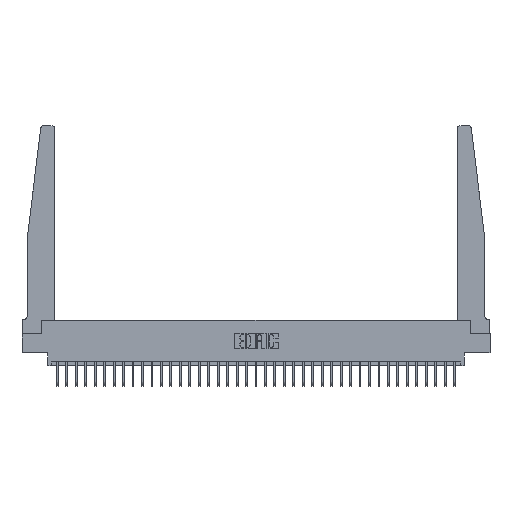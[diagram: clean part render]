
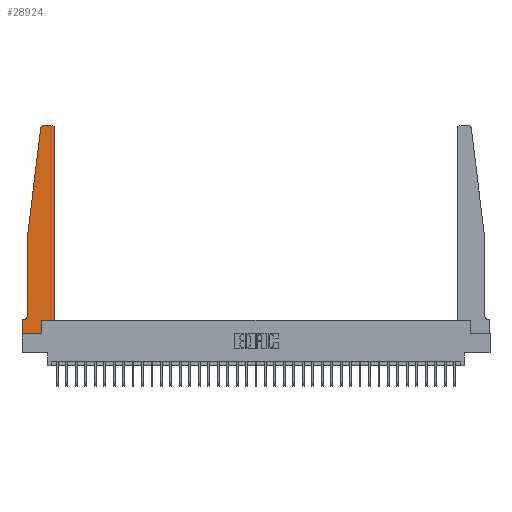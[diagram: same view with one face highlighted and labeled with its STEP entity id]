
A CAD part, top view. The second image highlights one B-rep face of the part: STEP entity #28924.
In plain terms, the highlighted planar face has unit normal (0, 0, 1).
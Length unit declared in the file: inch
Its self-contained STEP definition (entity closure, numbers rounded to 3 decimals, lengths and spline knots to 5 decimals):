
#155 = LINE ( 'NONE', #34775, #7327 ) ;
#225 = CARTESIAN_POINT ( 'NONE',  ( 0.27653, 2.72, 0.37 ) ) ;
#571 = CARTESIAN_POINT ( 'NONE',  ( 0.425, 0.18, 0.37 ) ) ;
#936 = VERTEX_POINT ( 'NONE', #23370 ) ;
#950 = CARTESIAN_POINT ( 'NONE',  ( 0.065, 1.25, 0.37 ) ) ;
#1851 = EDGE_CURVE ( 'NONE', #7147, #11979, #5981, .T. ) ;
#1907 = DIRECTION ( 'NONE',  ( 1., 0., 0. ) ) ;
#2014 = LINE ( 'NONE', #4502, #15001 ) ;
#2184 = VECTOR ( 'NONE', #29237, 39.37008 ) ;
#2485 = EDGE_CURVE ( 'NONE', #4802, #4737, #7721, .T. ) ;
#2605 = LINE ( 'NONE', #24413, #2184 ) ;
#3345 = CARTESIAN_POINT ( 'NONE',  ( 0.24675, 2.72367, 0.37 ) ) ;
#3614 = ORIENTED_EDGE ( 'NONE', *, *, #10190, .T. ) ;
#3928 = EDGE_CURVE ( 'NONE', #13896, #4141, #4807, .T. ) ;
#3960 = CARTESIAN_POINT ( 'NONE',  ( 0., 0.1875, 0.37 ) ) ;
#3990 = DIRECTION ( 'NONE',  ( 1., 0., 0. ) ) ;
#4141 = VERTEX_POINT ( 'NONE', #5384 ) ;
#4457 = EDGE_CURVE ( 'NONE', #21417, #7147, #25244, .T. ) ;
#4487 = CARTESIAN_POINT ( 'NONE',  ( 0.25, 2.75, 0.37 ) ) ;
#4502 = CARTESIAN_POINT ( 'NONE',  ( 0., 0., 0.37 ) ) ;
#4632 = EDGE_CURVE ( 'NONE', #936, #11196, #155, .T. ) ;
#4737 = VERTEX_POINT ( 'NONE', #3345 ) ;
#4747 = LINE ( 'NONE', #20705, #18385 ) ;
#4802 = VERTEX_POINT ( 'NONE', #26220 ) ;
#4807 = CIRCLE ( 'NONE', #7709, 0.03 ) ;
#5384 = CARTESIAN_POINT ( 'NONE',  ( 0.395, 2.75, 0.37 ) ) ;
#5981 = CIRCLE ( 'NONE', #29217, 0.05 ) ;
#6317 = CARTESIAN_POINT ( 'NONE',  ( 0.065, 0.1875, 0.37 ) ) ;
#7110 = FACE_OUTER_BOUND ( 'NONE', #29035, .T. ) ;
#7147 = VERTEX_POINT ( 'NONE', #27066 ) ;
#7327 = VECTOR ( 'NONE', #10977, 39.37008 ) ;
#7356 = CARTESIAN_POINT ( 'NONE',  ( 0.425, 0.18, 0.37 ) ) ;
#7709 = AXIS2_PLACEMENT_3D ( 'NONE', #28301, #19953, #3990 ) ;
#7721 = CIRCLE ( 'NONE', #27564, 0.03 ) ;
#7745 = DIRECTION ( 'NONE',  ( -0.122, -0.992, 0. ) ) ;
#8095 = CARTESIAN_POINT ( 'NONE',  ( 0.2605, 0.18, 0.37 ) ) ;
#8152 = ORIENTED_EDGE ( 'NONE', *, *, #18287, .T. ) ;
#8573 = DIRECTION ( 'NONE',  ( 0., 0., 1. ) ) ;
#8608 = DIRECTION ( 'NONE',  ( 0., -1., 0. ) ) ;
#9162 = DIRECTION ( 'NONE',  ( -1., 0., 0. ) ) ;
#10190 = EDGE_CURVE ( 'NONE', #4141, #4802, #28793, .T. ) ;
#10977 = DIRECTION ( 'NONE',  ( 0., 1., 0. ) ) ;
#11060 = EDGE_CURVE ( 'NONE', #4737, #21417, #4747, .T. ) ;
#11196 = VERTEX_POINT ( 'NONE', #8095 ) ;
#11979 = VERTEX_POINT ( 'NONE', #34951 ) ;
#12315 = VECTOR ( 'NONE', #32215, 39.37008 ) ;
#12773 = DIRECTION ( 'NONE',  ( 0., 0., 1. ) ) ;
#12938 = PLANE ( 'NONE',  #25368 ) ;
#13176 = EDGE_CURVE ( 'NONE', #29767, #936, #2014, .T. ) ;
#13896 = VERTEX_POINT ( 'NONE', #20019 ) ;
#14528 = EDGE_CURVE ( 'NONE', #30293, #29767, #24033, .T. ) ;
#15001 = VECTOR ( 'NONE', #15121, 39.37008 ) ;
#15121 = DIRECTION ( 'NONE',  ( 1., 0., 0. ) ) ;
#15223 = CARTESIAN_POINT ( 'NONE',  ( 0.015, 0.2375, 0.37 ) ) ;
#15998 = VECTOR ( 'NONE', #22579, 39.37008 ) ;
#16246 = ORIENTED_EDGE ( 'NONE', *, *, #13176, .T. ) ;
#16930 = VECTOR ( 'NONE', #9162, 39.37008 ) ;
#17140 = ORIENTED_EDGE ( 'NONE', *, *, #14528, .T. ) ;
#17893 = DIRECTION ( 'NONE',  ( 1., 0., 0. ) ) ;
#18287 = EDGE_CURVE ( 'NONE', #11979, #30293, #33663, .T. ) ;
#18385 = VECTOR ( 'NONE', #7745, 39.37008 ) ;
#18909 = ORIENTED_EDGE ( 'NONE', *, *, #2485, .T. ) ;
#19895 = LINE ( 'NONE', #571, #12315 ) ;
#19953 = DIRECTION ( 'NONE',  ( 0., 0., 1. ) ) ;
#20019 = CARTESIAN_POINT ( 'NONE',  ( 0.425, 2.72, 0.37 ) ) ;
#20705 = CARTESIAN_POINT ( 'NONE',  ( 0.065, 1.25, 0.37 ) ) ;
#21166 = ORIENTED_EDGE ( 'NONE', *, *, #4457, .T. ) ;
#21417 = VERTEX_POINT ( 'NONE', #22123 ) ;
#22123 = CARTESIAN_POINT ( 'NONE',  ( 0.065, 1.25, 0.37 ) ) ;
#22579 = DIRECTION ( 'NONE',  ( -1., 0., 0. ) ) ;
#23370 = CARTESIAN_POINT ( 'NONE',  ( 0.2605, 0., 0.37 ) ) ;
#23760 = CARTESIAN_POINT ( 'NONE',  ( 0., 0.1875, 0.37 ) ) ;
#24033 = LINE ( 'NONE', #27054, #30444 ) ;
#24413 = CARTESIAN_POINT ( 'NONE',  ( 0.425, 0.18, 0.37 ) ) ;
#24534 = ORIENTED_EDGE ( 'NONE', *, *, #4632, .T. ) ;
#25244 = LINE ( 'NONE', #950, #34325 ) ;
#25280 = ORIENTED_EDGE ( 'NONE', *, *, #29470, .T. ) ;
#25368 = AXIS2_PLACEMENT_3D ( 'NONE', #23760, #12773, #17893 ) ;
#25893 = EDGE_CURVE ( 'NONE', #11196, #28571, #19895, .T. ) ;
#26072 = DIRECTION ( 'NONE',  ( -1., 0., 0. ) ) ;
#26220 = CARTESIAN_POINT ( 'NONE',  ( 0.27653, 2.75, 0.37 ) ) ;
#27054 = CARTESIAN_POINT ( 'NONE',  ( 0., 0., 0.37 ) ) ;
#27066 = CARTESIAN_POINT ( 'NONE',  ( 0.065, 0.2375, 0.37 ) ) ;
#27564 = AXIS2_PLACEMENT_3D ( 'NONE', #225, #8573, #1907 ) ;
#28301 = CARTESIAN_POINT ( 'NONE',  ( 0.395, 2.72, 0.37 ) ) ;
#28571 = VERTEX_POINT ( 'NONE', #7356 ) ;
#28575 = DIRECTION ( 'NONE',  ( 0., -1., 0. ) ) ;
#28793 = LINE ( 'NONE', #4487, #15998 ) ;
#28821 = ORIENTED_EDGE ( 'NONE', *, *, #11060, .T. ) ;
#28844 = CARTESIAN_POINT ( 'NONE',  ( 0., 0., 0.37 ) ) ;
#28924 = ADVANCED_FACE ( 'NONE', ( #7110 ), #12938, .T. ) ;
#29035 = EDGE_LOOP ( 'NONE', ( #3614, #18909, #28821, #21166, #30619, #8152, #17140, #16246, #24534, #31237, #25280, #32713 ) ) ;
#29217 = AXIS2_PLACEMENT_3D ( 'NONE', #15223, #31421, #26072 ) ;
#29237 = DIRECTION ( 'NONE',  ( 0., 1., 0. ) ) ;
#29470 = EDGE_CURVE ( 'NONE', #28571, #13896, #2605, .T. ) ;
#29767 = VERTEX_POINT ( 'NONE', #28844 ) ;
#30293 = VERTEX_POINT ( 'NONE', #3960 ) ;
#30444 = VECTOR ( 'NONE', #8608, 39.37008 ) ;
#30619 = ORIENTED_EDGE ( 'NONE', *, *, #1851, .T. ) ;
#31237 = ORIENTED_EDGE ( 'NONE', *, *, #25893, .T. ) ;
#31421 = DIRECTION ( 'NONE',  ( 0., 0., -1. ) ) ;
#32215 = DIRECTION ( 'NONE',  ( 1., 0., 0. ) ) ;
#32713 = ORIENTED_EDGE ( 'NONE', *, *, #3928, .T. ) ;
#33663 = LINE ( 'NONE', #6317, #16930 ) ;
#34325 = VECTOR ( 'NONE', #28575, 39.37008 ) ;
#34775 = CARTESIAN_POINT ( 'NONE',  ( 0.2605, 0.18, 0.37 ) ) ;
#34951 = CARTESIAN_POINT ( 'NONE',  ( 0.015, 0.1875, 0.37 ) ) ;
